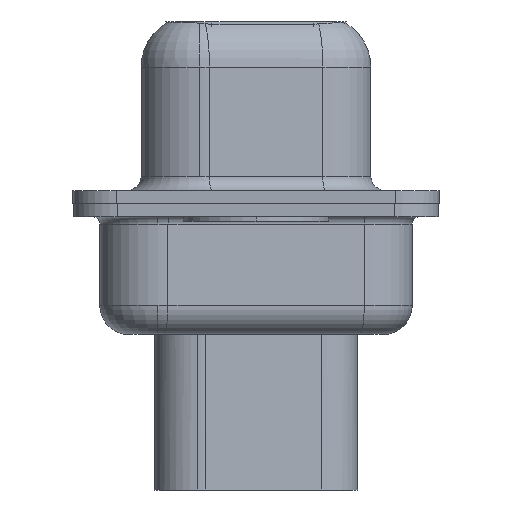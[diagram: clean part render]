
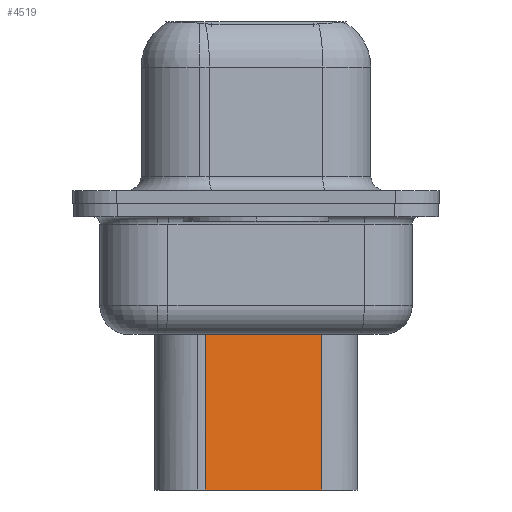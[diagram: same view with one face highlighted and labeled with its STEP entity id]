
A CAD part, left-side view. The second image highlights one B-rep face of the part: STEP entity #4519.
In plain terms, the highlighted planar face has unit normal (-0.985, -0.174, 0).
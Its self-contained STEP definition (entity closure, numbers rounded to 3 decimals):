
#135 = EDGE_CURVE ( 'NONE', #14861, #8790, #14977, .T. ) ;
#827 = CARTESIAN_POINT ( 'NONE',  ( 4.509, 1.74, -3.975 ) ) ;
#1008 = LINE ( 'NONE', #6271, #14047 ) ;
#1313 = VERTEX_POINT ( 'NONE', #827 ) ;
#1461 = VECTOR ( 'NONE', #11038, 1000. ) ;
#1952 = LINE ( 'NONE', #15177, #5977 ) ;
#3072 = VECTOR ( 'NONE', #4271, 1000. ) ;
#3223 = CARTESIAN_POINT ( 'NONE',  ( 4.509, 1.74, -9.85 ) ) ;
#3349 = CARTESIAN_POINT ( 'NONE',  ( 4.509, 1.74, -3.1 ) ) ;
#3460 = VERTEX_POINT ( 'NONE', #12908 ) ;
#4271 = DIRECTION ( 'NONE',  ( 0., 0., -1. ) ) ;
#4519 = ADVANCED_FACE ( 'NONE', ( #10994 ), #5682, .T. ) ;
#4751 = EDGE_CURVE ( 'NONE', #3460, #14861, #1008, .T. ) ;
#4836 = EDGE_CURVE ( 'NONE', #1313, #8790, #10632, .T. ) ;
#5575 = CARTESIAN_POINT ( 'NONE',  ( 4.509, 1.74, -3.1 ) ) ;
#5682 = PLANE ( 'NONE',  #7735 ) ;
#5943 = DIRECTION ( 'NONE',  ( 0.174, -0.985, 0. ) ) ;
#5977 = VECTOR ( 'NONE', #6440, 1000. ) ;
#6271 = CARTESIAN_POINT ( 'NONE',  ( 5.214, -2.26, -3.1 ) ) ;
#6440 = DIRECTION ( 'NONE',  ( -0.174, 0.985, 0. ) ) ;
#7234 = DIRECTION ( 'NONE',  ( -0.985, -0.174, 0. ) ) ;
#7402 = EDGE_CURVE ( 'NONE', #3460, #1313, #1952, .T. ) ;
#7735 = AXIS2_PLACEMENT_3D ( 'NONE', #3349, #7234, #5943 ) ;
#8790 = VERTEX_POINT ( 'NONE', #12176 ) ;
#9712 = EDGE_LOOP ( 'NONE', ( #13804, #12977, #13878, #13863 ) ) ;
#10632 = LINE ( 'NONE', #5575, #3072 ) ;
#10994 = FACE_OUTER_BOUND ( 'NONE', #9712, .T. ) ;
#11038 = DIRECTION ( 'NONE',  ( -0.174, 0.985, 0. ) ) ;
#11490 = DIRECTION ( 'NONE',  ( 0., 0., -1. ) ) ;
#12176 = CARTESIAN_POINT ( 'NONE',  ( 4.509, 1.74, -9.85 ) ) ;
#12908 = CARTESIAN_POINT ( 'NONE',  ( 5.214, -2.26, -3.975 ) ) ;
#12977 = ORIENTED_EDGE ( 'NONE', *, *, #7402, .T. ) ;
#13804 = ORIENTED_EDGE ( 'NONE', *, *, #4751, .F. ) ;
#13863 = ORIENTED_EDGE ( 'NONE', *, *, #135, .F. ) ;
#13878 = ORIENTED_EDGE ( 'NONE', *, *, #4836, .T. ) ;
#14047 = VECTOR ( 'NONE', #11490, 1000. ) ;
#14861 = VERTEX_POINT ( 'NONE', #16576 ) ;
#14977 = LINE ( 'NONE', #3223, #1461 ) ;
#15177 = CARTESIAN_POINT ( 'NONE',  ( 4.338, 2.709, -3.975 ) ) ;
#16576 = CARTESIAN_POINT ( 'NONE',  ( 5.214, -2.26, -9.85 ) ) ;
